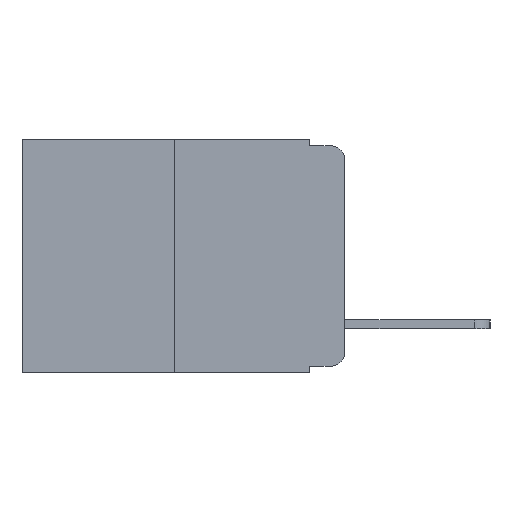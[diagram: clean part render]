
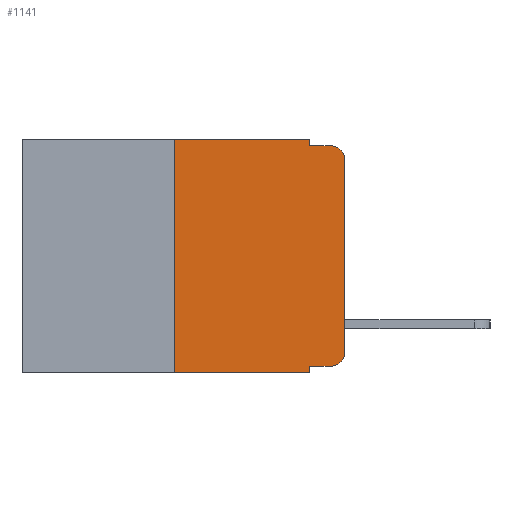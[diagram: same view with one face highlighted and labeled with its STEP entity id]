
A CAD part, left-side view. The second image highlights one B-rep face of the part: STEP entity #1141.
In plain terms, the highlighted planar face has unit normal (-1, 0, 0).
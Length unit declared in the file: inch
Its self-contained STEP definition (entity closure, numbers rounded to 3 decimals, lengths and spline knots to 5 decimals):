
#115 = EDGE_LOOP ( 'NONE', ( #12009, #7504, #12354, #2344, #10140, #8620, #546, #5665, #7180, #6003 ) ) ;
#213 = VERTEX_POINT ( 'NONE', #11459 ) ;
#361 = CARTESIAN_POINT ( 'NONE',  ( 0., 0.02, -0.03 ) ) ;
#390 = DIRECTION ( 'NONE',  ( 0., -1., 0. ) ) ;
#513 = LINE ( 'NONE', #11476, #11822 ) ;
#542 = EDGE_CURVE ( 'NONE', #5182, #4482, #3128, .T. ) ;
#546 = ORIENTED_EDGE ( 'NONE', *, *, #10711, .T. ) ;
#829 = DIRECTION ( 'NONE',  ( 0., 0., -1. ) ) ;
#1141 = ADVANCED_FACE ( 'NONE', ( #3953 ), #4920, .F. ) ;
#1475 = DIRECTION ( 'NONE',  ( 0., 0., 1. ) ) ;
#1699 = EDGE_CURVE ( 'NONE', #4482, #9039, #2386, .T. ) ;
#1714 = CARTESIAN_POINT ( 'NONE',  ( 0., 0.051, 0. ) ) ;
#1724 = CARTESIAN_POINT ( 'NONE',  ( 0., 0., -0.313 ) ) ;
#1778 = DIRECTION ( 'NONE',  ( 0., 0., -1. ) ) ;
#2331 = EDGE_CURVE ( 'NONE', #4083, #13338, #10677, .T. ) ;
#2344 = ORIENTED_EDGE ( 'NONE', *, *, #3149, .F. ) ;
#2382 = CARTESIAN_POINT ( 'NONE',  ( 0., 0.051, 0. ) ) ;
#2386 = CIRCLE ( 'NONE', #10277, 0.02 ) ;
#2567 = CARTESIAN_POINT ( 'NONE',  ( 0., 0.051, -0.333 ) ) ;
#2585 = CARTESIAN_POINT ( 'NONE',  ( 0., 0.25, 0. ) ) ;
#2764 = VECTOR ( 'NONE', #6212, 39.37008 ) ;
#2835 = CARTESIAN_POINT ( 'NONE',  ( 0., 0.051, 0. ) ) ;
#3128 = LINE ( 'NONE', #11413, #11329 ) ;
#3149 = EDGE_CURVE ( 'NONE', #9778, #12580, #10987, .T. ) ;
#3252 = AXIS2_PLACEMENT_3D ( 'NONE', #8060, #3815, #8101 ) ;
#3616 = DIRECTION ( 'NONE',  ( 0., -1., 0. ) ) ;
#3655 = VECTOR ( 'NONE', #390, 39.37008 ) ;
#3771 = EDGE_CURVE ( 'NONE', #13338, #9778, #513, .T. ) ;
#3815 = DIRECTION ( 'NONE',  ( -1., 0., 0. ) ) ;
#3953 = FACE_OUTER_BOUND ( 'NONE', #115, .T. ) ;
#4083 = VERTEX_POINT ( 'NONE', #8705 ) ;
#4482 = VERTEX_POINT ( 'NONE', #6248 ) ;
#4699 = VECTOR ( 'NONE', #3616, 39.37008 ) ;
#4920 = PLANE ( 'NONE',  #10811 ) ;
#4961 = CARTESIAN_POINT ( 'NONE',  ( 0., 0.473, 0. ) ) ;
#5182 = VERTEX_POINT ( 'NONE', #1724 ) ;
#5228 = LINE ( 'NONE', #2835, #11259 ) ;
#5305 = CARTESIAN_POINT ( 'NONE',  ( 0., 0.02, -0.01 ) ) ;
#5310 = EDGE_CURVE ( 'NONE', #10940, #213, #5228, .T. ) ;
#5321 = EDGE_CURVE ( 'NONE', #10023, #5182, #13406, .T. ) ;
#5642 = CARTESIAN_POINT ( 'NONE',  ( 0., 0.051, -0.01 ) ) ;
#5665 = ORIENTED_EDGE ( 'NONE', *, *, #5310, .F. ) ;
#5679 = DIRECTION ( 'NONE',  ( 0., 0., -1. ) ) ;
#6003 = ORIENTED_EDGE ( 'NONE', *, *, #5321, .T. ) ;
#6212 = DIRECTION ( 'NONE',  ( 0., -1., 0. ) ) ;
#6248 = CARTESIAN_POINT ( 'NONE',  ( 0., 0., -0.03 ) ) ;
#7180 = ORIENTED_EDGE ( 'NONE', *, *, #12768, .T. ) ;
#7389 = EDGE_CURVE ( 'NONE', #12580, #9039, #12187, .T. ) ;
#7493 = DIRECTION ( 'NONE',  ( -1., 0., 0. ) ) ;
#7504 = ORIENTED_EDGE ( 'NONE', *, *, #1699, .T. ) ;
#7563 = CARTESIAN_POINT ( 'NONE',  ( 0., 0.051, -0.01 ) ) ;
#7812 = VECTOR ( 'NONE', #5679, 39.37008 ) ;
#8060 = CARTESIAN_POINT ( 'NONE',  ( 0., 0.02, -0.313 ) ) ;
#8101 = DIRECTION ( 'NONE',  ( 0., 0., -1. ) ) ;
#8620 = ORIENTED_EDGE ( 'NONE', *, *, #2331, .F. ) ;
#8705 = CARTESIAN_POINT ( 'NONE',  ( 0., 0.25, -0.343 ) ) ;
#9039 = VERTEX_POINT ( 'NONE', #5305 ) ;
#9095 = LINE ( 'NONE', #11540, #2764 ) ;
#9778 = VERTEX_POINT ( 'NONE', #2382 ) ;
#9928 = DIRECTION ( 'NONE',  ( 1., 0., 0. ) ) ;
#10023 = VERTEX_POINT ( 'NONE', #11279 ) ;
#10067 = DIRECTION ( 'NONE',  ( 0., 0., -1. ) ) ;
#10140 = ORIENTED_EDGE ( 'NONE', *, *, #3771, .F. ) ;
#10277 = AXIS2_PLACEMENT_3D ( 'NONE', #361, #7493, #829 ) ;
#10348 = VECTOR ( 'NONE', #1475, 39.37008 ) ;
#10581 = DIRECTION ( 'NONE',  ( 0., 0., 1. ) ) ;
#10580 = DIRECTION ( 'NONE',  ( 0., -1., 0. ) ) ;
#10677 = LINE ( 'NONE', #2585, #10348 ) ;
#10711 = EDGE_CURVE ( 'NONE', #4083, #213, #9095, .T. ) ;
#10811 = AXIS2_PLACEMENT_3D ( 'NONE', #4961, #9928, #10067 ) ;
#10856 = CARTESIAN_POINT ( 'NONE',  ( 0., 0.051, -0.333 ) ) ;
#10940 = VERTEX_POINT ( 'NONE', #10856 ) ;
#10987 = LINE ( 'NONE', #1714, #7812 ) ;
#11259 = VECTOR ( 'NONE', #1778, 39.37008 ) ;
#11279 = CARTESIAN_POINT ( 'NONE',  ( 0., 0.02, -0.333 ) ) ;
#11329 = VECTOR ( 'NONE', #10581, 39.37008 ) ;
#11413 = CARTESIAN_POINT ( 'NONE',  ( 0., 0., 0. ) ) ;
#11459 = CARTESIAN_POINT ( 'NONE',  ( 0., 0.051, -0.343 ) ) ;
#11476 = CARTESIAN_POINT ( 'NONE',  ( 0., 0.473, 0. ) ) ;
#11540 = CARTESIAN_POINT ( 'NONE',  ( 0., 0.473, -0.343 ) ) ;
#11822 = VECTOR ( 'NONE', #10580, 39.37008 ) ;
#12009 = ORIENTED_EDGE ( 'NONE', *, *, #542, .T. ) ;
#12154 = CARTESIAN_POINT ( 'NONE',  ( 0., 0.25, 0. ) ) ;
#12187 = LINE ( 'NONE', #5642, #3655 ) ;
#12354 = ORIENTED_EDGE ( 'NONE', *, *, #7389, .F. ) ;
#12580 = VERTEX_POINT ( 'NONE', #7563 ) ;
#12768 = EDGE_CURVE ( 'NONE', #10940, #10023, #13228, .T. ) ;
#13228 = LINE ( 'NONE', #2567, #4699 ) ;
#13338 = VERTEX_POINT ( 'NONE', #12154 ) ;
#13406 = CIRCLE ( 'NONE', #3252, 0.02 ) ;
